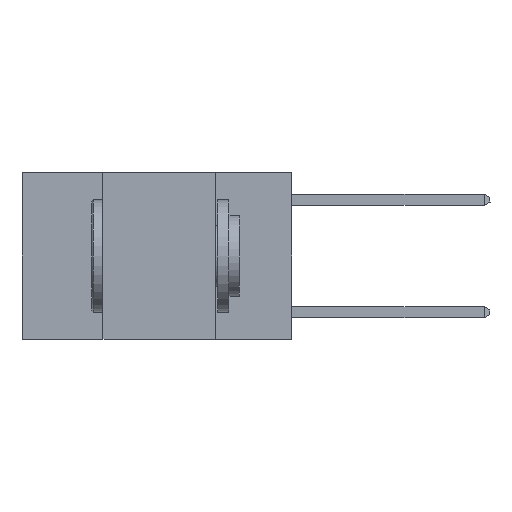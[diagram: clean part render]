
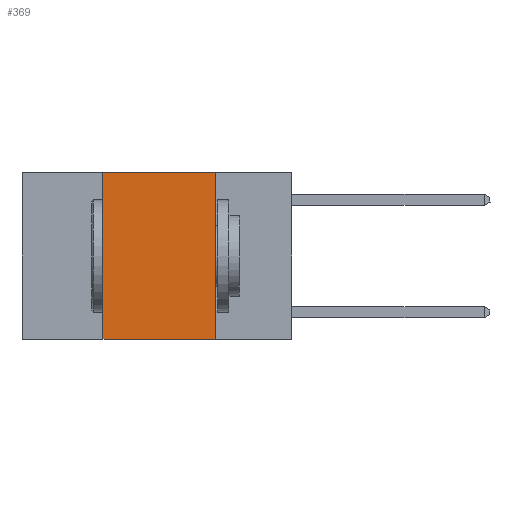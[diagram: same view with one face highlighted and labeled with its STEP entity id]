
A CAD part, left-side view. The second image highlights one B-rep face of the part: STEP entity #369.
In plain terms, the highlighted planar face has unit normal (-1, 0, 0).
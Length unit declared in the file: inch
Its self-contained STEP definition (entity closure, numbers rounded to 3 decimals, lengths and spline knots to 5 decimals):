
#233 = AXIS2_PLACEMENT_3D ( 'NONE', #13354, #5682, #17520 ) ;
#369 = ADVANCED_FACE ( 'NONE', ( #8461 ), #14044, .F. ) ;
#600 = EDGE_LOOP ( 'NONE', ( #4934, #6073, #1569, #2024 ) ) ;
#1383 = LINE ( 'NONE', #3855, #9978 ) ;
#1471 = VERTEX_POINT ( 'NONE', #13785 ) ;
#1569 = ORIENTED_EDGE ( 'NONE', *, *, #21479, .F. ) ;
#2024 = ORIENTED_EDGE ( 'NONE', *, *, #20382, .T. ) ;
#3855 = CARTESIAN_POINT ( 'NONE',  ( 0., 0.17, 0. ) ) ;
#4272 = CARTESIAN_POINT ( 'NONE',  ( 0., 0.6, 0. ) ) ;
#4934 = ORIENTED_EDGE ( 'NONE', *, *, #8158, .F. ) ;
#5416 = VERTEX_POINT ( 'NONE', #19120 ) ;
#5682 = DIRECTION ( 'NONE',  ( 1., 0., 0. ) ) ;
#6073 = ORIENTED_EDGE ( 'NONE', *, *, #17926, .F. ) ;
#7868 = VERTEX_POINT ( 'NONE', #15159 ) ;
#8158 = EDGE_CURVE ( 'NONE', #9846, #5416, #1383, .T. ) ;
#8461 = FACE_OUTER_BOUND ( 'NONE', #600, .T. ) ;
#9210 = LINE ( 'NONE', #9428, #17776 ) ;
#9428 = CARTESIAN_POINT ( 'NONE',  ( 0., 0.6, -0.37 ) ) ;
#9846 = VERTEX_POINT ( 'NONE', #15182 ) ;
#9978 = VECTOR ( 'NONE', #15827, 39.37008 ) ;
#10798 = DIRECTION ( 'NONE',  ( 0., 0., 1. ) ) ;
#11130 = DIRECTION ( 'NONE',  ( 0., -1., 0. ) ) ;
#12917 = DIRECTION ( 'NONE',  ( 0., -1., 0. ) ) ;
#13204 = VECTOR ( 'NONE', #10798, 39.37008 ) ;
#13354 = CARTESIAN_POINT ( 'NONE',  ( 0., 0.6, 0. ) ) ;
#13785 = CARTESIAN_POINT ( 'NONE',  ( 0., 0.42, -0.37 ) ) ;
#14044 = PLANE ( 'NONE',  #233 ) ;
#15159 = CARTESIAN_POINT ( 'NONE',  ( 0., 0.42, 0. ) ) ;
#15182 = CARTESIAN_POINT ( 'NONE',  ( 0., 0.17, 0. ) ) ;
#15827 = DIRECTION ( 'NONE',  ( 0., 0., -1. ) ) ;
#16343 = VECTOR ( 'NONE', #12917, 39.37008 ) ;
#17520 = DIRECTION ( 'NONE',  ( 0., 0., -1. ) ) ;
#17776 = VECTOR ( 'NONE', #11130, 39.37008 ) ;
#17926 = EDGE_CURVE ( 'NONE', #7868, #9846, #20765, .T. ) ;
#19120 = CARTESIAN_POINT ( 'NONE',  ( 0., 0.17, -0.37 ) ) ;
#20382 = EDGE_CURVE ( 'NONE', #1471, #5416, #9210, .T. ) ;
#20765 = LINE ( 'NONE', #4272, #16343 ) ;
#20929 = CARTESIAN_POINT ( 'NONE',  ( 0., 0.42, 0. ) ) ;
#21479 = EDGE_CURVE ( 'NONE', #1471, #7868, #21609, .T. ) ;
#21609 = LINE ( 'NONE', #20929, #13204 ) ;
